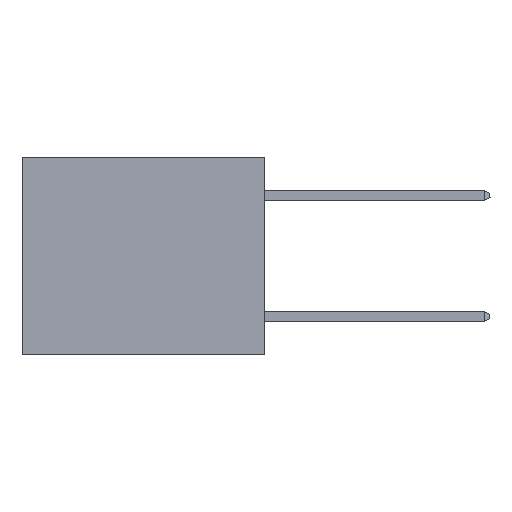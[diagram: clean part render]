
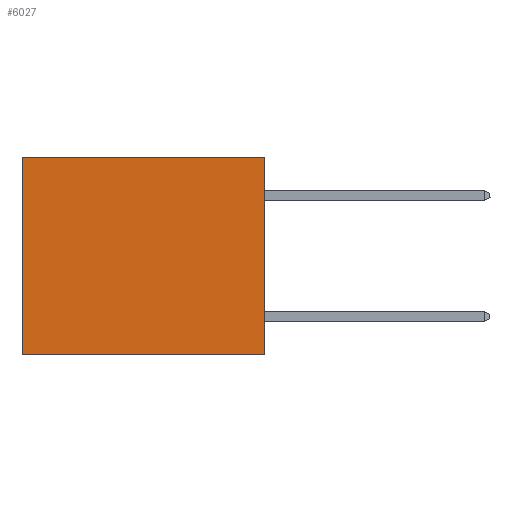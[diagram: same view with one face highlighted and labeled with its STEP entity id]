
A CAD part, left-side view. The second image highlights one B-rep face of the part: STEP entity #6027.
In plain terms, the highlighted planar face has unit normal (-1, 0, 0).
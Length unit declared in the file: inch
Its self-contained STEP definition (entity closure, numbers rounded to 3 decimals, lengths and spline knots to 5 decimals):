
#759 = AXIS2_PLACEMENT_3D ( 'NONE', #16978, #11011, #12848 ) ;
#891 = VERTEX_POINT ( 'NONE', #24375 ) ;
#1409 = CARTESIAN_POINT ( 'NONE',  ( 0.3165, 0., -0.49 ) ) ;
#1767 = CARTESIAN_POINT ( 'NONE',  ( 0.3165, 0.6, -0.49 ) ) ;
#2413 = CARTESIAN_POINT ( 'NONE',  ( 0.3165, 0., 0. ) ) ;
#2591 = EDGE_CURVE ( 'NONE', #16448, #21035, #7743, .T. ) ;
#2679 = CARTESIAN_POINT ( 'NONE',  ( 0.3165, 0., 0. ) ) ;
#3171 = ORIENTED_EDGE ( 'NONE', *, *, #20054, .F. ) ;
#3485 = DIRECTION ( 'NONE',  ( 0., 0., -1. ) ) ;
#4208 = PLANE ( 'NONE',  #759 ) ;
#5878 = EDGE_LOOP ( 'NONE', ( #9158, #3171, #25990, #19627 ) ) ;
#6027 = ADVANCED_FACE ( 'NONE', ( #24482 ), #4208, .F. ) ;
#7743 = LINE ( 'NONE', #24392, #11012 ) ;
#9158 = ORIENTED_EDGE ( 'NONE', *, *, #12421, .T. ) ;
#9808 = VERTEX_POINT ( 'NONE', #25926 ) ;
#11011 = DIRECTION ( 'NONE',  ( 1., 0., 0. ) ) ;
#11012 = VECTOR ( 'NONE', #3485, 39.37008 ) ;
#11143 = DIRECTION ( 'NONE',  ( 0., 1., 0. ) ) ;
#11745 = CARTESIAN_POINT ( 'NONE',  ( 0.3165, 0., -0.49 ) ) ;
#12001 = VECTOR ( 'NONE', #11143, 39.37008 ) ;
#12421 = EDGE_CURVE ( 'NONE', #9808, #891, #20316, .T. ) ;
#12560 = VECTOR ( 'NONE', #23773, 39.37008 ) ;
#12848 = DIRECTION ( 'NONE',  ( 0., 0., -1. ) ) ;
#13642 = DIRECTION ( 'NONE',  ( 0., 0., -1. ) ) ;
#16448 = VERTEX_POINT ( 'NONE', #2413 ) ;
#16978 = CARTESIAN_POINT ( 'NONE',  ( 0.3165, 0., -0.49 ) ) ;
#18021 = VECTOR ( 'NONE', #13642, 39.37008 ) ;
#19627 = ORIENTED_EDGE ( 'NONE', *, *, #23850, .T. ) ;
#20054 = EDGE_CURVE ( 'NONE', #21035, #891, #23126, .T. ) ;
#20316 = LINE ( 'NONE', #1767, #18021 ) ;
#21035 = VERTEX_POINT ( 'NONE', #11745 ) ;
#23126 = LINE ( 'NONE', #1409, #12560 ) ;
#23773 = DIRECTION ( 'NONE',  ( 0., 1., 0. ) ) ;
#23850 = EDGE_CURVE ( 'NONE', #16448, #9808, #26856, .T. ) ;
#24375 = CARTESIAN_POINT ( 'NONE',  ( 0.3165, 0.6, -0.49 ) ) ;
#24392 = CARTESIAN_POINT ( 'NONE',  ( 0.3165, 0., -0.49 ) ) ;
#24482 = FACE_OUTER_BOUND ( 'NONE', #5878, .T. ) ;
#25926 = CARTESIAN_POINT ( 'NONE',  ( 0.3165, 0.6, 0. ) ) ;
#25990 = ORIENTED_EDGE ( 'NONE', *, *, #2591, .F. ) ;
#26856 = LINE ( 'NONE', #2679, #12001 ) ;
